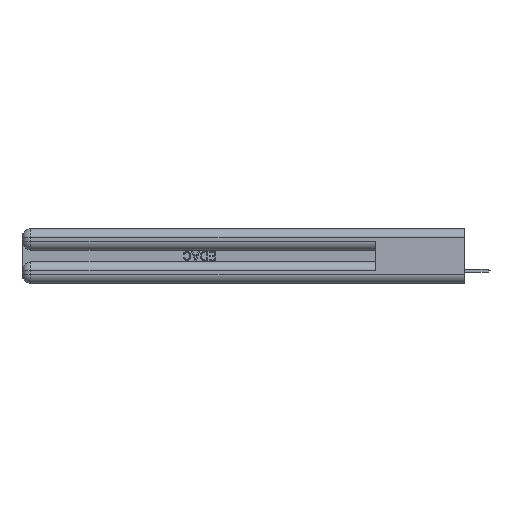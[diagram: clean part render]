
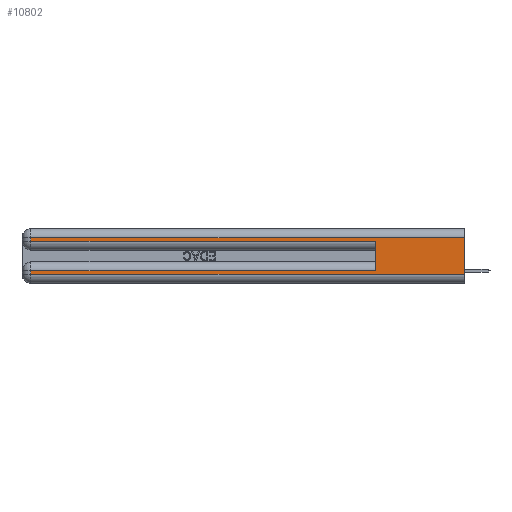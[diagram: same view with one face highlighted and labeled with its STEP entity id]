
A CAD part, left-side view. The second image highlights one B-rep face of the part: STEP entity #10802.
In plain terms, the highlighted planar face has unit normal (-1, 0, 0).
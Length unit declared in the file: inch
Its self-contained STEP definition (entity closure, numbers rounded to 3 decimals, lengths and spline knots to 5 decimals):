
#587 = VECTOR ( 'NONE', #22213, 39.37008 ) ;
#1327 = VECTOR ( 'NONE', #10114, 39.37008 ) ;
#2085 = CARTESIAN_POINT ( 'NONE',  ( 0., 0., 0.06 ) ) ;
#2469 = ORIENTED_EDGE ( 'NONE', *, *, #29476, .F. ) ;
#2684 = ORIENTED_EDGE ( 'NONE', *, *, #34468, .T. ) ;
#4021 = LINE ( 'NONE', #37922, #34893 ) ;
#4817 = EDGE_LOOP ( 'NONE', ( #2469, #38014, #19792, #11354, #15037, #18942, #2684, #25213 ) ) ;
#5666 = DIRECTION ( 'NONE',  ( 0., 1., 0. ) ) ;
#5701 = VERTEX_POINT ( 'NONE', #14995 ) ;
#6555 = VECTOR ( 'NONE', #11372, 39.37008 ) ;
#6565 = VERTEX_POINT ( 'NONE', #27020 ) ;
#6715 = EDGE_CURVE ( 'NONE', #27265, #26670, #18971, .T. ) ;
#7076 = LINE ( 'NONE', #30094, #11048 ) ;
#9621 = DIRECTION ( 'NONE',  ( 0., 0., -1. ) ) ;
#9937 = CARTESIAN_POINT ( 'NONE',  ( 0., 0., 0.06 ) ) ;
#10114 = DIRECTION ( 'NONE',  ( 0., 0., 1. ) ) ;
#10802 = ADVANCED_FACE ( 'NONE', ( #28124 ), #30365, .F. ) ;
#11048 = VECTOR ( 'NONE', #17375, 39.37008 ) ;
#11247 = CARTESIAN_POINT ( 'NONE',  ( 0., 0., 0.37 ) ) ;
#11354 = ORIENTED_EDGE ( 'NONE', *, *, #6715, .T. ) ;
#11372 = DIRECTION ( 'NONE',  ( 0., -1., 0. ) ) ;
#13276 = VERTEX_POINT ( 'NONE', #9937 ) ;
#13330 = VECTOR ( 'NONE', #9621, 39.37008 ) ;
#14995 = CARTESIAN_POINT ( 'NONE',  ( 0., 2.94, 0.31 ) ) ;
#15037 = ORIENTED_EDGE ( 'NONE', *, *, #35104, .F. ) ;
#16209 = VECTOR ( 'NONE', #33366, 39.37008 ) ;
#17375 = DIRECTION ( 'NONE',  ( 0., 0., -1. ) ) ;
#17639 = CARTESIAN_POINT ( 'NONE',  ( 0., 2.94, 0.085 ) ) ;
#18942 = ORIENTED_EDGE ( 'NONE', *, *, #32769, .T. ) ;
#18971 = LINE ( 'NONE', #33641, #6555 ) ;
#19792 = ORIENTED_EDGE ( 'NONE', *, *, #21795, .T. ) ;
#20823 = CARTESIAN_POINT ( 'NONE',  ( 0., 2.94, 0.37 ) ) ;
#21282 = DIRECTION ( 'NONE',  ( 1., 0., 0. ) ) ;
#21362 = LINE ( 'NONE', #34561, #13330 ) ;
#21795 = EDGE_CURVE ( 'NONE', #5701, #27265, #33194, .T. ) ;
#22213 = DIRECTION ( 'NONE',  ( 0., 1., 0. ) ) ;
#22644 = CARTESIAN_POINT ( 'NONE',  ( 0., 0.6, 0.145 ) ) ;
#24725 = CARTESIAN_POINT ( 'NONE',  ( 0., 0., 0.31 ) ) ;
#24816 = LINE ( 'NONE', #22644, #1327 ) ;
#25213 = ORIENTED_EDGE ( 'NONE', *, *, #32396, .T. ) ;
#25628 = CARTESIAN_POINT ( 'NONE',  ( 0., 2.94, 0.06 ) ) ;
#25825 = CARTESIAN_POINT ( 'NONE',  ( 0., 2.94, 0.285 ) ) ;
#26670 = VERTEX_POINT ( 'NONE', #39537 ) ;
#27020 = CARTESIAN_POINT ( 'NONE',  ( 0., 0.6, 0.085 ) ) ;
#27265 = VERTEX_POINT ( 'NONE', #25825 ) ;
#28124 = FACE_OUTER_BOUND ( 'NONE', #4817, .T. ) ;
#29476 = EDGE_CURVE ( 'NONE', #31917, #13276, #7076, .T. ) ;
#30094 = CARTESIAN_POINT ( 'NONE',  ( 0., 0., 0.37 ) ) ;
#30302 = EDGE_CURVE ( 'NONE', #31917, #5701, #4021, .T. ) ;
#30365 = PLANE ( 'NONE',  #38549 ) ;
#30873 = VERTEX_POINT ( 'NONE', #25628 ) ;
#31063 = LINE ( 'NONE', #41149, #587 ) ;
#31917 = VERTEX_POINT ( 'NONE', #24725 ) ;
#32396 = EDGE_CURVE ( 'NONE', #30873, #13276, #39994, .T. ) ;
#32543 = VECTOR ( 'NONE', #33655, 39.37008 ) ;
#32769 = EDGE_CURVE ( 'NONE', #6565, #40312, #31063, .T. ) ;
#33194 = LINE ( 'NONE', #20823, #16209 ) ;
#33366 = DIRECTION ( 'NONE',  ( 0., 0., -1. ) ) ;
#33641 = CARTESIAN_POINT ( 'NONE',  ( 0., 0., 0.285 ) ) ;
#33655 = DIRECTION ( 'NONE',  ( 0., -1., 0. ) ) ;
#34468 = EDGE_CURVE ( 'NONE', #40312, #30873, #21362, .T. ) ;
#34561 = CARTESIAN_POINT ( 'NONE',  ( 0., 2.94, 0.37 ) ) ;
#34893 = VECTOR ( 'NONE', #5666, 39.37008 ) ;
#35104 = EDGE_CURVE ( 'NONE', #6565, #26670, #24816, .T. ) ;
#37922 = CARTESIAN_POINT ( 'NONE',  ( 0., 0., 0.31 ) ) ;
#38014 = ORIENTED_EDGE ( 'NONE', *, *, #30302, .T. ) ;
#38549 = AXIS2_PLACEMENT_3D ( 'NONE', #11247, #21282, #39919 ) ;
#39537 = CARTESIAN_POINT ( 'NONE',  ( 0., 0.6, 0.285 ) ) ;
#39919 = DIRECTION ( 'NONE',  ( 0., 0., -1. ) ) ;
#39994 = LINE ( 'NONE', #2085, #32543 ) ;
#40312 = VERTEX_POINT ( 'NONE', #17639 ) ;
#41149 = CARTESIAN_POINT ( 'NONE',  ( 0., 0., 0.085 ) ) ;
